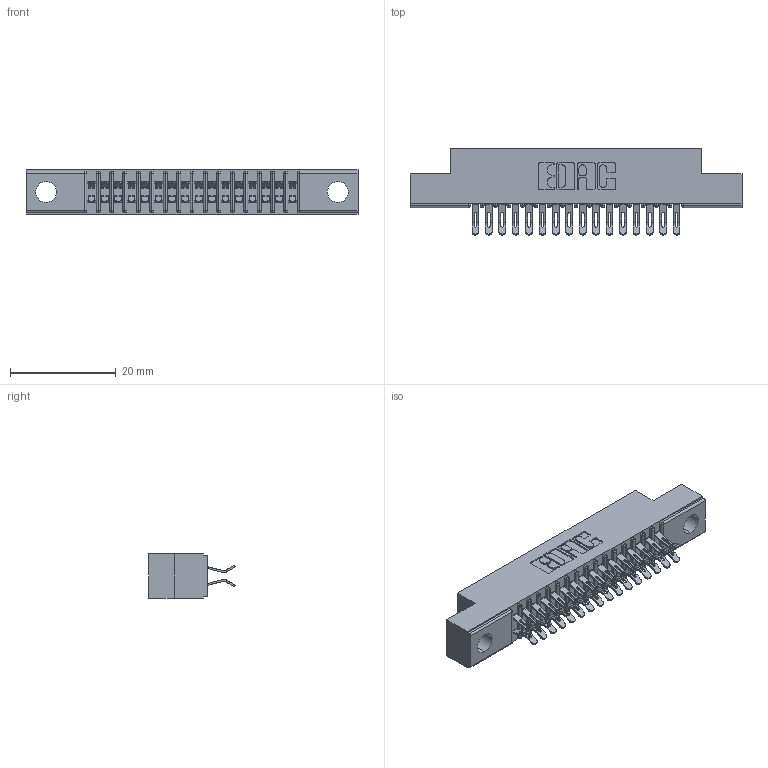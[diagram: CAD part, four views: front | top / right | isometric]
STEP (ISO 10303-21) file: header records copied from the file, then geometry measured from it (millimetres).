
FILE_DESCRIPTION (( 'STEP AP203' ), '1' );
FILE_NAME ('341-032-555-204.STEP', '2018-08-06T21:05:32', ( '' ), ( '' ), 'SwSTEP 2.0', 'SolidWorks 2016', '' );
FILE_SCHEMA (( 'CONFIG_CONTROL_DESIGN' ));
Length unit declared in the file: inch
Products named in the file (3): 341 Part_.156 (3.96) Dia Mounting Holes; 341-292-001_341-292-155; 341-032-555-204
Assembly tree (33 placements, depth 2):
  341-032-555-204
    341 Part_.156 (3.96) Dia Mounting Holes
    341-292-001_341-292-155  x32
Bounding box: 62.87 x 16.31 x 8.38 mm (x, y, z)
Volume: 3530.1 mm3; surface area: 7150.5 mm2
Topology: 33 solids, 33 shells, 2626 faces, 7824 edges, 5094 vertices
Faces by surface type: plane 1426, cylinder 1136, sphere 34, torus 30
Entity records: 23715 total; most frequent: CARTESIAN_POINT 3964, ORIENTED_EDGE 3924, DIRECTION 3848, EDGE_CURVE 1962, VECTOR 1548, LINE 1548, VERTEX_POINT 1250, AXIS2_PLACEMENT_3D 1150
